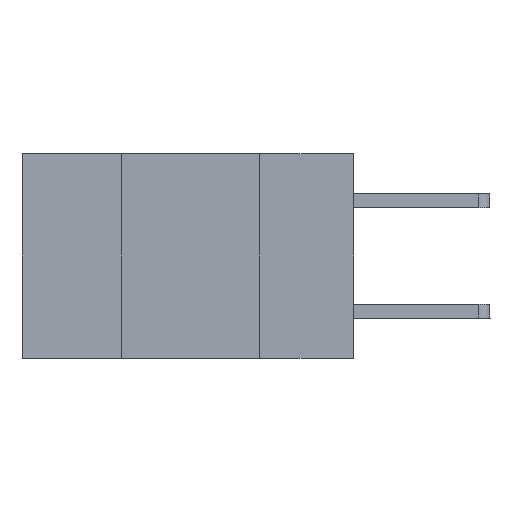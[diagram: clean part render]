
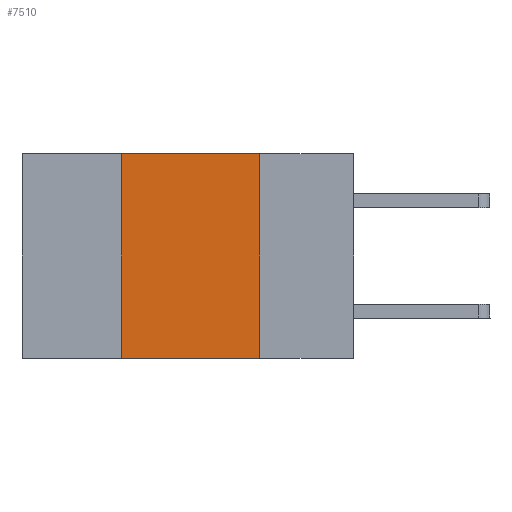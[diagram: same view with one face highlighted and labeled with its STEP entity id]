
A CAD part, left-side view. The second image highlights one B-rep face of the part: STEP entity #7510.
In plain terms, the highlighted planar face has unit normal (-1, 0, 0).
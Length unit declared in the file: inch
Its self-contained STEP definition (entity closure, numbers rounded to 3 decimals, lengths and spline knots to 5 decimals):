
#440 = VERTEX_POINT ( 'NONE', #7365 ) ;
#548 = LINE ( 'NONE', #10454, #11034 ) ;
#688 = EDGE_CURVE ( 'NONE', #9832, #10478, #9004, .T. ) ;
#1268 = VERTEX_POINT ( 'NONE', #6528 ) ;
#1396 = CARTESIAN_POINT ( 'NONE',  ( 0., 0.17, -0.37 ) ) ;
#1819 = DIRECTION ( 'NONE',  ( 1., 0., 0. ) ) ;
#2957 = FACE_OUTER_BOUND ( 'NONE', #12706, .T. ) ;
#3023 = DIRECTION ( 'NONE',  ( 0., -1., 0. ) ) ;
#3126 = EDGE_CURVE ( 'NONE', #1268, #10478, #10079, .T. ) ;
#3540 = CARTESIAN_POINT ( 'NONE',  ( 0., 0.17, 0. ) ) ;
#3554 = CARTESIAN_POINT ( 'NONE',  ( 0., 0.6, -0.37 ) ) ;
#4557 = VECTOR ( 'NONE', #3023, 39.37008 ) ;
#4956 = CARTESIAN_POINT ( 'NONE',  ( 0., 0.6, 0. ) ) ;
#5466 = VECTOR ( 'NONE', #10065, 39.37008 ) ;
#6119 = ORIENTED_EDGE ( 'NONE', *, *, #6943, .F. ) ;
#6129 = ORIENTED_EDGE ( 'NONE', *, *, #11506, .F. ) ;
#6528 = CARTESIAN_POINT ( 'NONE',  ( 0., 0.42, -0.37 ) ) ;
#6943 = EDGE_CURVE ( 'NONE', #1268, #440, #548, .T. ) ;
#7144 = DIRECTION ( 'NONE',  ( 0., -1., 0. ) ) ;
#7365 = CARTESIAN_POINT ( 'NONE',  ( 0., 0.42, 0. ) ) ;
#7510 = ADVANCED_FACE ( 'NONE', ( #2957 ), #11490, .F. ) ;
#7984 = ORIENTED_EDGE ( 'NONE', *, *, #3126, .T. ) ;
#8472 = CARTESIAN_POINT ( 'NONE',  ( 0., 0.6, 0. ) ) ;
#9004 = LINE ( 'NONE', #3540, #5466 ) ;
#9168 = DIRECTION ( 'NONE',  ( 0., 0., 1. ) ) ;
#9832 = VERTEX_POINT ( 'NONE', #14101 ) ;
#10065 = DIRECTION ( 'NONE',  ( 0., 0., -1. ) ) ;
#10079 = LINE ( 'NONE', #3554, #11209 ) ;
#10454 = CARTESIAN_POINT ( 'NONE',  ( 0., 0.42, 0. ) ) ;
#10478 = VERTEX_POINT ( 'NONE', #1396 ) ;
#10620 = LINE ( 'NONE', #8472, #4557 ) ;
#10624 = DIRECTION ( 'NONE',  ( 0., 0., -1. ) ) ;
#11034 = VECTOR ( 'NONE', #9168, 39.37008 ) ;
#11209 = VECTOR ( 'NONE', #7144, 39.37008 ) ;
#11490 = PLANE ( 'NONE',  #12648 ) ;
#11506 = EDGE_CURVE ( 'NONE', #440, #9832, #10620, .T. ) ;
#12437 = ORIENTED_EDGE ( 'NONE', *, *, #688, .F. ) ;
#12648 = AXIS2_PLACEMENT_3D ( 'NONE', #4956, #1819, #10624 ) ;
#12706 = EDGE_LOOP ( 'NONE', ( #12437, #6129, #6119, #7984 ) ) ;
#14101 = CARTESIAN_POINT ( 'NONE',  ( 0., 0.17, 0. ) ) ;
